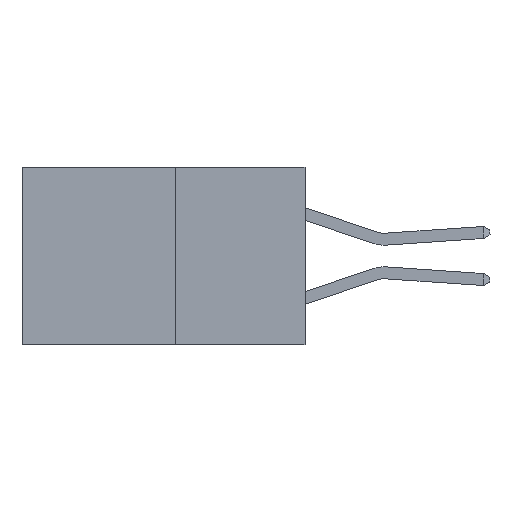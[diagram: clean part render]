
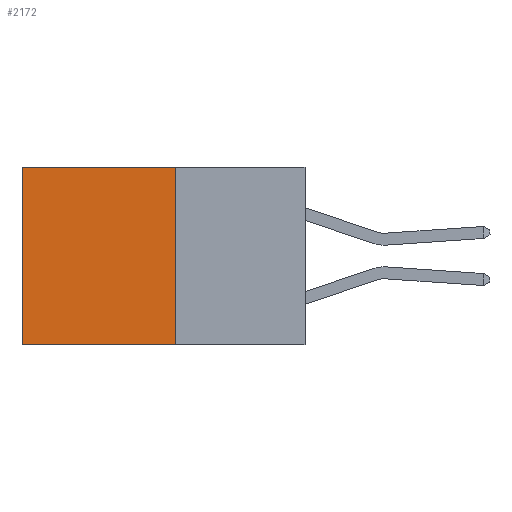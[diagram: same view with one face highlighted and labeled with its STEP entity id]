
A CAD part, left-side view. The second image highlights one B-rep face of the part: STEP entity #2172.
In plain terms, the highlighted planar face has unit normal (-1, 0, 0).
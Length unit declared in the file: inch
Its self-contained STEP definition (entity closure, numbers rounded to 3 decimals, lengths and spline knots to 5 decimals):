
#236 = CARTESIAN_POINT ( 'NONE',  ( 0.277, 0.59, -0.37 ) ) ;
#600 = LINE ( 'NONE', #7223, #4670 ) ;
#679 = CARTESIAN_POINT ( 'NONE',  ( 0.277, 0.27, -0.37 ) ) ;
#1002 = DIRECTION ( 'NONE',  ( 0., 0., -1. ) ) ;
#1138 = FACE_OUTER_BOUND ( 'NONE', #9991, .T. ) ;
#1204 = LINE ( 'NONE', #8188, #5198 ) ;
#1730 = DIRECTION ( 'NONE',  ( 1., 0., 0. ) ) ;
#2172 = ADVANCED_FACE ( 'NONE', ( #1138 ), #9032, .F. ) ;
#2180 = DIRECTION ( 'NONE',  ( 0., 0., -1. ) ) ;
#2379 = DIRECTION ( 'NONE',  ( 0., 0., -1. ) ) ;
#2972 = EDGE_CURVE ( 'NONE', #5459, #5392, #5803, .T. ) ;
#3569 = VECTOR ( 'NONE', #9957, 39.37008 ) ;
#4391 = CARTESIAN_POINT ( 'NONE',  ( 0.277, 0.27, 0. ) ) ;
#4509 = VERTEX_POINT ( 'NONE', #679 ) ;
#4668 = AXIS2_PLACEMENT_3D ( 'NONE', #9941, #1730, #1002 ) ;
#4670 = VECTOR ( 'NONE', #2379, 39.37008 ) ;
#5181 = ORIENTED_EDGE ( 'NONE', *, *, #9876, .F. ) ;
#5198 = VECTOR ( 'NONE', #8998, 39.37008 ) ;
#5392 = VERTEX_POINT ( 'NONE', #236 ) ;
#5426 = ORIENTED_EDGE ( 'NONE', *, *, #7504, .T. ) ;
#5459 = VERTEX_POINT ( 'NONE', #10060 ) ;
#5803 = LINE ( 'NONE', #7000, #8332 ) ;
#7000 = CARTESIAN_POINT ( 'NONE',  ( 0.277, 0.59, -0.37 ) ) ;
#7223 = CARTESIAN_POINT ( 'NONE',  ( 0.277, 0.27, -0.37 ) ) ;
#7432 = ORIENTED_EDGE ( 'NONE', *, *, #8671, .F. ) ;
#7504 = EDGE_CURVE ( 'NONE', #9372, #5459, #7967, .T. ) ;
#7967 = LINE ( 'NONE', #9144, #3569 ) ;
#8188 = CARTESIAN_POINT ( 'NONE',  ( 0.277, 0.27, -0.37 ) ) ;
#8332 = VECTOR ( 'NONE', #2180, 39.37008 ) ;
#8671 = EDGE_CURVE ( 'NONE', #9372, #4509, #600, .T. ) ;
#8998 = DIRECTION ( 'NONE',  ( 0., 1., 0. ) ) ;
#9032 = PLANE ( 'NONE',  #4668 ) ;
#9144 = CARTESIAN_POINT ( 'NONE',  ( 0.277, 0.27, 0. ) ) ;
#9332 = ORIENTED_EDGE ( 'NONE', *, *, #2972, .T. ) ;
#9372 = VERTEX_POINT ( 'NONE', #4391 ) ;
#9876 = EDGE_CURVE ( 'NONE', #4509, #5392, #1204, .T. ) ;
#9941 = CARTESIAN_POINT ( 'NONE',  ( 0.277, 0.27, -0.37 ) ) ;
#9957 = DIRECTION ( 'NONE',  ( 0., 1., 0. ) ) ;
#9991 = EDGE_LOOP ( 'NONE', ( #9332, #5181, #7432, #5426 ) ) ;
#10060 = CARTESIAN_POINT ( 'NONE',  ( 0.277, 0.59, 0. ) ) ;
